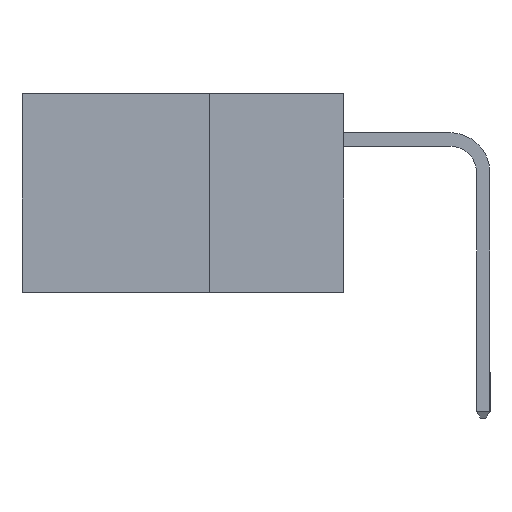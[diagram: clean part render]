
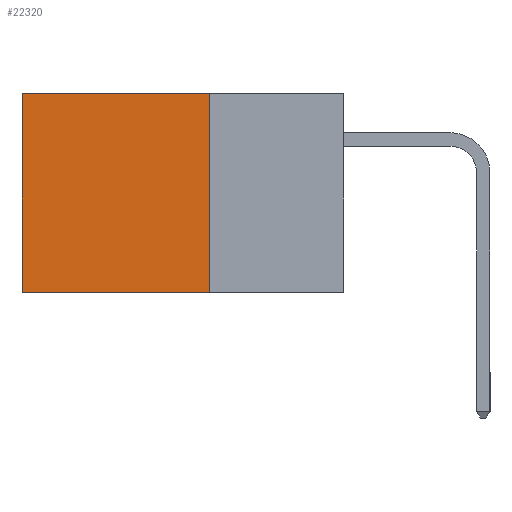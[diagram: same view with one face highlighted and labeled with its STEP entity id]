
A CAD part, left-side view. The second image highlights one B-rep face of the part: STEP entity #22320.
In plain terms, the highlighted planar face has unit normal (-1, 0, 0).
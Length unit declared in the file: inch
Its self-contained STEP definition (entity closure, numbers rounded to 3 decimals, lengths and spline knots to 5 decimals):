
#968 = CARTESIAN_POINT ( 'NONE',  ( 0.298, 0.25, 0. ) ) ;
#976 = LINE ( 'NONE', #968, #6156 ) ;
#2769 = LINE ( 'NONE', #17401, #21953 ) ;
#3218 = AXIS2_PLACEMENT_3D ( 'NONE', #5444, #15805, #10768 ) ;
#3444 = CARTESIAN_POINT ( 'NONE',  ( 0.298, 0.25, 0. ) ) ;
#4190 = CARTESIAN_POINT ( 'NONE',  ( 0.298, 0.25, 0. ) ) ;
#4225 = LINE ( 'NONE', #22588, #17085 ) ;
#5292 = VERTEX_POINT ( 'NONE', #7953 ) ;
#5444 = CARTESIAN_POINT ( 'NONE',  ( 0.298, 0.25, 0. ) ) ;
#5658 = VERTEX_POINT ( 'NONE', #15709 ) ;
#6156 = VECTOR ( 'NONE', #16578, 39.37008 ) ;
#6475 = ORIENTED_EDGE ( 'NONE', *, *, #10776, .F. ) ;
#6932 = DIRECTION ( 'NONE',  ( 0., 0., -1. ) ) ;
#7784 = EDGE_CURVE ( 'NONE', #5658, #5292, #2769, .T. ) ;
#7953 = CARTESIAN_POINT ( 'NONE',  ( 0.298, 0.6, -0.37 ) ) ;
#8702 = ORIENTED_EDGE ( 'NONE', *, *, #7784, .F. ) ;
#8767 = PLANE ( 'NONE',  #3218 ) ;
#8851 = DIRECTION ( 'NONE',  ( 0., 1., 0. ) ) ;
#9791 = EDGE_CURVE ( 'NONE', #15617, #19262, #976, .T. ) ;
#10670 = EDGE_CURVE ( 'NONE', #19262, #5292, #4225, .T. ) ;
#10768 = DIRECTION ( 'NONE',  ( 0., 0., -1. ) ) ;
#10776 = EDGE_CURVE ( 'NONE', #15617, #5658, #17910, .T. ) ;
#11389 = VECTOR ( 'NONE', #17217, 39.37008 ) ;
#15118 = ORIENTED_EDGE ( 'NONE', *, *, #9791, .T. ) ;
#15514 = FACE_OUTER_BOUND ( 'NONE', #16533, .T. ) ;
#15617 = VERTEX_POINT ( 'NONE', #4190 ) ;
#15709 = CARTESIAN_POINT ( 'NONE',  ( 0.298, 0.25, -0.37 ) ) ;
#15805 = DIRECTION ( 'NONE',  ( 1., 0., 0. ) ) ;
#16533 = EDGE_LOOP ( 'NONE', ( #21643, #8702, #6475, #15118 ) ) ;
#16578 = DIRECTION ( 'NONE',  ( 0., 1., 0. ) ) ;
#17085 = VECTOR ( 'NONE', #6932, 39.37008 ) ;
#17217 = DIRECTION ( 'NONE',  ( 0., 0., -1. ) ) ;
#17401 = CARTESIAN_POINT ( 'NONE',  ( 0.298, 0.25, -0.37 ) ) ;
#17910 = LINE ( 'NONE', #3444, #11389 ) ;
#18400 = CARTESIAN_POINT ( 'NONE',  ( 0.298, 0.6, 0. ) ) ;
#19262 = VERTEX_POINT ( 'NONE', #18400 ) ;
#21643 = ORIENTED_EDGE ( 'NONE', *, *, #10670, .T. ) ;
#21953 = VECTOR ( 'NONE', #8851, 39.37008 ) ;
#22320 = ADVANCED_FACE ( 'NONE', ( #15514 ), #8767, .F. ) ;
#22588 = CARTESIAN_POINT ( 'NONE',  ( 0.298, 0.6, 0. ) ) ;
